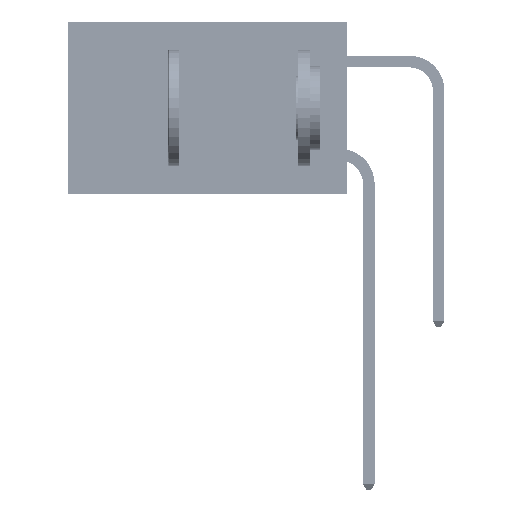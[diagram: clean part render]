
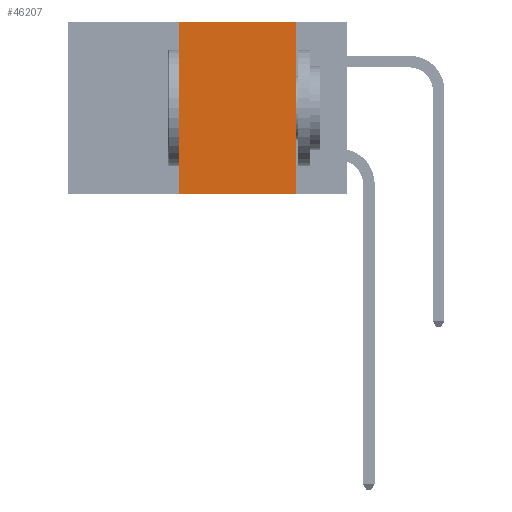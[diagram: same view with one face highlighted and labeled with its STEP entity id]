
A CAD part, left-side view. The second image highlights one B-rep face of the part: STEP entity #46207.
In plain terms, the highlighted planar face has unit normal (-1, 0, 0).
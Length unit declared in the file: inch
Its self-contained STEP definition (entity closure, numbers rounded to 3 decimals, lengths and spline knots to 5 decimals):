
#705 = VECTOR ( 'NONE', #8395, 39.37008 ) ;
#2147 = EDGE_CURVE ( 'NONE', #38996, #5109, #27857, .T. ) ;
#2365 = DIRECTION ( 'NONE',  ( 0., -1., 0. ) ) ;
#5109 = VERTEX_POINT ( 'NONE', #34427 ) ;
#6111 = CARTESIAN_POINT ( 'NONE',  ( 0., 0.11, 0. ) ) ;
#6180 = CARTESIAN_POINT ( 'NONE',  ( 0., 0.36, -0.37 ) ) ;
#6263 = DIRECTION ( 'NONE',  ( 0., 0., 1. ) ) ;
#7499 = DIRECTION ( 'NONE',  ( 0., 0., -1. ) ) ;
#7650 = CARTESIAN_POINT ( 'NONE',  ( 0., 0.6, 0. ) ) ;
#8395 = DIRECTION ( 'NONE',  ( 0., -1., 0. ) ) ;
#8731 = VECTOR ( 'NONE', #6263, 39.37008 ) ;
#9536 = CARTESIAN_POINT ( 'NONE',  ( 0., 0.36, 0. ) ) ;
#11278 = PLANE ( 'NONE',  #42815 ) ;
#13301 = LINE ( 'NONE', #31198, #8731 ) ;
#13665 = CARTESIAN_POINT ( 'NONE',  ( 0., 0.11, 0. ) ) ;
#13807 = VECTOR ( 'NONE', #34863, 39.37008 ) ;
#20895 = EDGE_CURVE ( 'NONE', #37122, #5109, #43154, .T. ) ;
#21963 = DIRECTION ( 'NONE',  ( 1., 0., 0. ) ) ;
#24728 = ORIENTED_EDGE ( 'NONE', *, *, #20895, .T. ) ;
#27764 = CARTESIAN_POINT ( 'NONE',  ( 0., 0.6, -0.37 ) ) ;
#27857 = LINE ( 'NONE', #13665, #13807 ) ;
#29072 = VECTOR ( 'NONE', #2365, 39.37008 ) ;
#29907 = LINE ( 'NONE', #33523, #705 ) ;
#30072 = ORIENTED_EDGE ( 'NONE', *, *, #40476, .F. ) ;
#31198 = CARTESIAN_POINT ( 'NONE',  ( 0., 0.36, 0. ) ) ;
#31300 = ORIENTED_EDGE ( 'NONE', *, *, #36767, .F. ) ;
#33523 = CARTESIAN_POINT ( 'NONE',  ( 0., 0.6, 0. ) ) ;
#33979 = EDGE_LOOP ( 'NONE', ( #34650, #31300, #30072, #24728 ) ) ;
#34427 = CARTESIAN_POINT ( 'NONE',  ( 0., 0.11, -0.37 ) ) ;
#34556 = VERTEX_POINT ( 'NONE', #9536 ) ;
#34650 = ORIENTED_EDGE ( 'NONE', *, *, #2147, .F. ) ;
#34863 = DIRECTION ( 'NONE',  ( 0., 0., -1. ) ) ;
#36767 = EDGE_CURVE ( 'NONE', #34556, #38996, #29907, .T. ) ;
#37122 = VERTEX_POINT ( 'NONE', #6180 ) ;
#38309 = FACE_OUTER_BOUND ( 'NONE', #33979, .T. ) ;
#38996 = VERTEX_POINT ( 'NONE', #6111 ) ;
#40476 = EDGE_CURVE ( 'NONE', #37122, #34556, #13301, .T. ) ;
#42815 = AXIS2_PLACEMENT_3D ( 'NONE', #7650, #21963, #7499 ) ;
#43154 = LINE ( 'NONE', #27764, #29072 ) ;
#46207 = ADVANCED_FACE ( 'NONE', ( #38309 ), #11278, .F. ) ;
